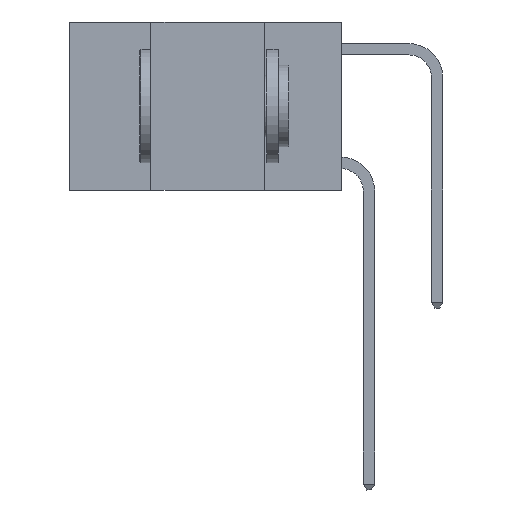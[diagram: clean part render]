
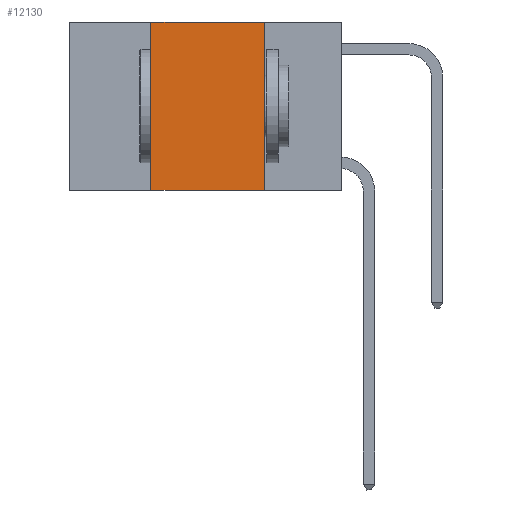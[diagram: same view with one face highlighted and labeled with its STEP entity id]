
A CAD part, left-side view. The second image highlights one B-rep face of the part: STEP entity #12130.
In plain terms, the highlighted planar face has unit normal (-1, 0, 0).
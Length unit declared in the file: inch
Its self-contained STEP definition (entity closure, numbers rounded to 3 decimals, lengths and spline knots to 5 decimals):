
#302 = VECTOR ( 'NONE', #6710, 39.37008 ) ;
#831 = CARTESIAN_POINT ( 'NONE',  ( 0., 0.6, 0. ) ) ;
#1349 = VERTEX_POINT ( 'NONE', #4134 ) ;
#1505 = CARTESIAN_POINT ( 'NONE',  ( 0., 0.17, 0. ) ) ;
#1801 = LINE ( 'NONE', #4909, #9044 ) ;
#1888 = DIRECTION ( 'NONE',  ( 0., -1., 0. ) ) ;
#2020 = CARTESIAN_POINT ( 'NONE',  ( 0., 0.6, -0.37 ) ) ;
#2440 = DIRECTION ( 'NONE',  ( 1., 0., 0. ) ) ;
#2612 = CARTESIAN_POINT ( 'NONE',  ( 0., 0.17, -0.37 ) ) ;
#2693 = ORIENTED_EDGE ( 'NONE', *, *, #7354, .T. ) ;
#2757 = CARTESIAN_POINT ( 'NONE',  ( 0., 0.17, 0. ) ) ;
#4134 = CARTESIAN_POINT ( 'NONE',  ( 0., 0.42, -0.37 ) ) ;
#4292 = PLANE ( 'NONE',  #5895 ) ;
#4432 = FACE_OUTER_BOUND ( 'NONE', #5203, .T. ) ;
#4712 = ORIENTED_EDGE ( 'NONE', *, *, #9258, .F. ) ;
#4787 = DIRECTION ( 'NONE',  ( 0., 0., 1. ) ) ;
#4909 = CARTESIAN_POINT ( 'NONE',  ( 0., 0.42, 0. ) ) ;
#5203 = EDGE_LOOP ( 'NONE', ( #9027, #4712, #12320, #2693 ) ) ;
#5895 = AXIS2_PLACEMENT_3D ( 'NONE', #8326, #2440, #10346 ) ;
#6710 = DIRECTION ( 'NONE',  ( 0., 0., -1. ) ) ;
#7354 = EDGE_CURVE ( 'NONE', #1349, #11382, #10772, .T. ) ;
#7695 = LINE ( 'NONE', #2757, #302 ) ;
#7967 = EDGE_CURVE ( 'NONE', #9608, #11382, #7695, .T. ) ;
#8326 = CARTESIAN_POINT ( 'NONE',  ( 0., 0.6, 0. ) ) ;
#8653 = DIRECTION ( 'NONE',  ( 0., -1., 0. ) ) ;
#8844 = LINE ( 'NONE', #831, #9009 ) ;
#8889 = VERTEX_POINT ( 'NONE', #9864 ) ;
#9009 = VECTOR ( 'NONE', #8653, 39.37008 ) ;
#9027 = ORIENTED_EDGE ( 'NONE', *, *, #7967, .F. ) ;
#9044 = VECTOR ( 'NONE', #4787, 39.37008 ) ;
#9258 = EDGE_CURVE ( 'NONE', #8889, #9608, #8844, .T. ) ;
#9608 = VERTEX_POINT ( 'NONE', #1505 ) ;
#9864 = CARTESIAN_POINT ( 'NONE',  ( 0., 0.42, 0. ) ) ;
#10162 = EDGE_CURVE ( 'NONE', #1349, #8889, #1801, .T. ) ;
#10346 = DIRECTION ( 'NONE',  ( 0., 0., -1. ) ) ;
#10772 = LINE ( 'NONE', #2020, #11040 ) ;
#11040 = VECTOR ( 'NONE', #1888, 39.37008 ) ;
#11382 = VERTEX_POINT ( 'NONE', #2612 ) ;
#12130 = ADVANCED_FACE ( 'NONE', ( #4432 ), #4292, .F. ) ;
#12320 = ORIENTED_EDGE ( 'NONE', *, *, #10162, .F. ) ;
